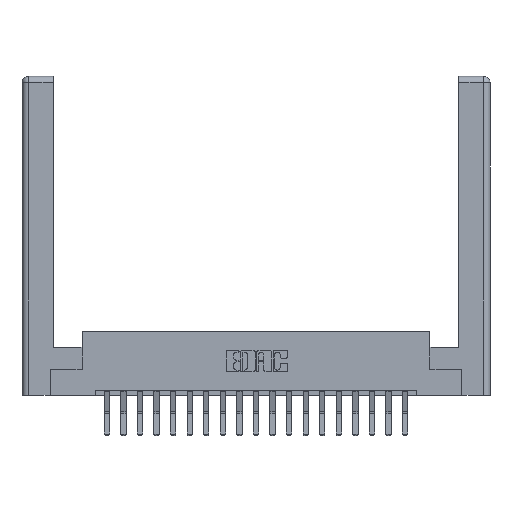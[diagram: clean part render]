
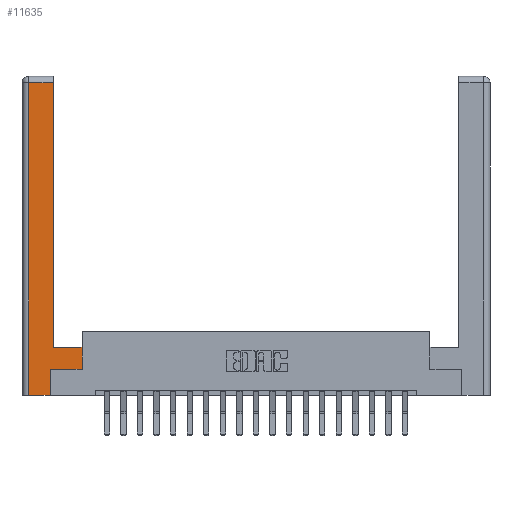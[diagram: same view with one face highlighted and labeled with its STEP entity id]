
A CAD part, top view. The second image highlights one B-rep face of the part: STEP entity #11635.
In plain terms, the highlighted planar face has unit normal (0, 0, 1).
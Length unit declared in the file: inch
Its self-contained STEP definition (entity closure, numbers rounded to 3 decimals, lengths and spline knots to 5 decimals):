
#230 = DIRECTION ( 'NONE',  ( 0., 1., 0. ) ) ;
#692 = VERTEX_POINT ( 'NONE', #2260 ) ;
#729 = EDGE_CURVE ( 'NONE', #18735, #10122, #17382, .T. ) ;
#842 = DIRECTION ( 'NONE',  ( -1., 0., 0. ) ) ;
#941 = CARTESIAN_POINT ( 'NONE',  ( 0.565, 0.245, 0. ) ) ;
#1018 = AXIS2_PLACEMENT_3D ( 'NONE', #14270, #9879, #842 ) ;
#1056 = ORIENTED_EDGE ( 'NONE', *, *, #16587, .T. ) ;
#2193 = VECTOR ( 'NONE', #11977, 39.37008 ) ;
#2260 = CARTESIAN_POINT ( 'NONE',  ( 0.265, 0.245, 0. ) ) ;
#2273 = LINE ( 'NONE', #3415, #19531 ) ;
#2528 = CARTESIAN_POINT ( 'NONE',  ( 0.265, 0., 0. ) ) ;
#2593 = EDGE_CURVE ( 'NONE', #692, #15110, #11558, .T. ) ;
#2939 = VECTOR ( 'NONE', #8975, 39.37008 ) ;
#3110 = EDGE_CURVE ( 'NONE', #19298, #11685, #13254, .T. ) ;
#3415 = CARTESIAN_POINT ( 'NONE',  ( 0.265, 0.245, 0. ) ) ;
#3689 = CARTESIAN_POINT ( 'NONE',  ( 0.295, 0.45, 0. ) ) ;
#4090 = VECTOR ( 'NONE', #7032, 39.37008 ) ;
#5665 = EDGE_LOOP ( 'NONE', ( #6884, #6666, #11837, #14364, #17268, #16985, #1056, #7958 ) ) ;
#5739 = EDGE_CURVE ( 'NONE', #18768, #19608, #18761, .T. ) ;
#6092 = LINE ( 'NONE', #19660, #18387 ) ;
#6469 = DIRECTION ( 'NONE',  ( 1., 0., 0. ) ) ;
#6666 = ORIENTED_EDGE ( 'NONE', *, *, #729, .T. ) ;
#6695 = CARTESIAN_POINT ( 'NONE',  ( 0.265, 0., 0. ) ) ;
#6884 = ORIENTED_EDGE ( 'NONE', *, *, #14376, .T. ) ;
#6946 = EDGE_CURVE ( 'NONE', #19608, #692, #2273, .T. ) ;
#6971 = CARTESIAN_POINT ( 'NONE',  ( 0.295, 3., 0. ) ) ;
#7032 = DIRECTION ( 'NONE',  ( -1., 0., 0. ) ) ;
#7103 = CARTESIAN_POINT ( 'NONE',  ( 0.0615, 2.94, 0. ) ) ;
#7681 = EDGE_CURVE ( 'NONE', #10122, #18768, #12568, .T. ) ;
#7958 = ORIENTED_EDGE ( 'NONE', *, *, #3110, .T. ) ;
#8082 = VECTOR ( 'NONE', #10617, 39.37008 ) ;
#8382 = CARTESIAN_POINT ( 'NONE',  ( 0.295, 2.94, 0. ) ) ;
#8975 = DIRECTION ( 'NONE',  ( 0., -1., 0. ) ) ;
#9615 = VECTOR ( 'NONE', #17986, 39.37008 ) ;
#9879 = DIRECTION ( 'NONE',  ( 0., 0., -1. ) ) ;
#9922 = VECTOR ( 'NONE', #6469, 39.37008 ) ;
#10090 = DIRECTION ( 'NONE',  ( 0., 1., 0. ) ) ;
#10122 = VERTEX_POINT ( 'NONE', #12226 ) ;
#10605 = LINE ( 'NONE', #6971, #9615 ) ;
#10617 = DIRECTION ( 'NONE',  ( -1., 0., 0. ) ) ;
#11558 = LINE ( 'NONE', #941, #2193 ) ;
#11604 = CARTESIAN_POINT ( 'NONE',  ( 0.0615, 0., 0. ) ) ;
#11635 = ADVANCED_FACE ( 'NONE', ( #20150 ), #14199, .F. ) ;
#11685 = VERTEX_POINT ( 'NONE', #3689 ) ;
#11821 = CARTESIAN_POINT ( 'NONE',  ( 0.565, 0.245, 0. ) ) ;
#11837 = ORIENTED_EDGE ( 'NONE', *, *, #7681, .T. ) ;
#11977 = DIRECTION ( 'NONE',  ( 1., 0., 0. ) ) ;
#12226 = CARTESIAN_POINT ( 'NONE',  ( 0.0615, 2.94, 0. ) ) ;
#12568 = LINE ( 'NONE', #16844, #2939 ) ;
#13254 = LINE ( 'NONE', #13640, #8082 ) ;
#13640 = CARTESIAN_POINT ( 'NONE',  ( 0.295, 0.45, 0. ) ) ;
#14199 = PLANE ( 'NONE',  #1018 ) ;
#14270 = CARTESIAN_POINT ( 'NONE',  ( 0., 0., 0. ) ) ;
#14364 = ORIENTED_EDGE ( 'NONE', *, *, #5739, .T. ) ;
#14376 = EDGE_CURVE ( 'NONE', #11685, #18735, #10605, .T. ) ;
#15110 = VERTEX_POINT ( 'NONE', #11821 ) ;
#16587 = EDGE_CURVE ( 'NONE', #15110, #19298, #6092, .T. ) ;
#16844 = CARTESIAN_POINT ( 'NONE',  ( 0.0615, 0., 0. ) ) ;
#16985 = ORIENTED_EDGE ( 'NONE', *, *, #2593, .T. ) ;
#17268 = ORIENTED_EDGE ( 'NONE', *, *, #6946, .T. ) ;
#17382 = LINE ( 'NONE', #7103, #4090 ) ;
#17986 = DIRECTION ( 'NONE',  ( 0., 1., 0. ) ) ;
#18380 = CARTESIAN_POINT ( 'NONE',  ( 0.565, 0.45, 0. ) ) ;
#18387 = VECTOR ( 'NONE', #10090, 39.37008 ) ;
#18735 = VERTEX_POINT ( 'NONE', #8382 ) ;
#18761 = LINE ( 'NONE', #6695, #9922 ) ;
#18768 = VERTEX_POINT ( 'NONE', #11604 ) ;
#19298 = VERTEX_POINT ( 'NONE', #18380 ) ;
#19531 = VECTOR ( 'NONE', #230, 39.37008 ) ;
#19608 = VERTEX_POINT ( 'NONE', #2528 ) ;
#19660 = CARTESIAN_POINT ( 'NONE',  ( 0.565, 0.45, 0. ) ) ;
#20150 = FACE_OUTER_BOUND ( 'NONE', #5665, .T. ) ;
